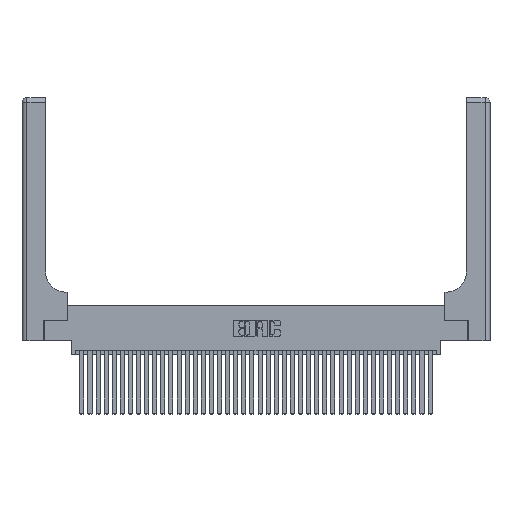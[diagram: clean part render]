
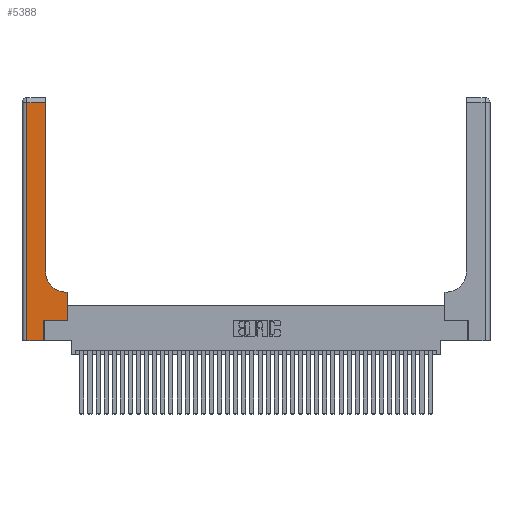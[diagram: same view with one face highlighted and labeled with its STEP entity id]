
A CAD part, top view. The second image highlights one B-rep face of the part: STEP entity #5388.
In plain terms, the highlighted planar face has unit normal (0, 0, 1).
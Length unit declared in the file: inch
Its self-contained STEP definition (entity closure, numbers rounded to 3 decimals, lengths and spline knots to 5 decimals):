
#55 = VERTEX_POINT ( 'NONE', #9593 ) ;
#679 = VERTEX_POINT ( 'NONE', #28018 ) ;
#1475 = VECTOR ( 'NONE', #24072, 39.37008 ) ;
#1845 = VERTEX_POINT ( 'NONE', #36134 ) ;
#2176 = VECTOR ( 'NONE', #4003, 39.37008 ) ;
#2212 = LINE ( 'NONE', #38274, #26557 ) ;
#4003 = DIRECTION ( 'NONE',  ( -1., 0., 0. ) ) ;
#5207 = ORIENTED_EDGE ( 'NONE', *, *, #17527, .T. ) ;
#5388 = ADVANCED_FACE ( 'NONE', ( #31855 ), #8118, .F. ) ;
#5506 = LINE ( 'NONE', #39268, #29762 ) ;
#7099 = VERTEX_POINT ( 'NONE', #28311 ) ;
#7922 = DIRECTION ( 'NONE',  ( 0., 1., 0. ) ) ;
#8118 = PLANE ( 'NONE',  #24441 ) ;
#8122 = ORIENTED_EDGE ( 'NONE', *, *, #33617, .T. ) ;
#8871 = CARTESIAN_POINT ( 'NONE',  ( 0.5415, 0.6, 0.37 ) ) ;
#9434 = DIRECTION ( 'NONE',  ( 0., -1., 0. ) ) ;
#9593 = CARTESIAN_POINT ( 'NONE',  ( 0.269, 0.25, 0.37 ) ) ;
#9673 = LINE ( 'NONE', #33059, #1475 ) ;
#10085 = DIRECTION ( 'NONE',  ( 0., 0., -1. ) ) ;
#10752 = DIRECTION ( 'NONE',  ( 0., 1., 0. ) ) ;
#11184 = DIRECTION ( 'NONE',  ( 0., 0., -1. ) ) ;
#11329 = LINE ( 'NONE', #19222, #2176 ) ;
#11651 = VERTEX_POINT ( 'NONE', #26555 ) ;
#12263 = CARTESIAN_POINT ( 'NONE',  ( 0.2915, 0.6, 0.37 ) ) ;
#12870 = CARTESIAN_POINT ( 'NONE',  ( 0.269, 0., 0.37 ) ) ;
#13168 = LINE ( 'NONE', #25882, #22160 ) ;
#13370 = ORIENTED_EDGE ( 'NONE', *, *, #27678, .T. ) ;
#14698 = VECTOR ( 'NONE', #33447, 39.37008 ) ;
#15318 = EDGE_CURVE ( 'NONE', #38560, #55, #30430, .T. ) ;
#15475 = CARTESIAN_POINT ( 'NONE',  ( 0.06, 3., 0.37 ) ) ;
#16254 = ORIENTED_EDGE ( 'NONE', *, *, #18850, .T. ) ;
#17061 = EDGE_CURVE ( 'NONE', #7099, #11651, #2212, .T. ) ;
#17527 = EDGE_CURVE ( 'NONE', #11651, #38305, #11329, .T. ) ;
#18408 = AXIS2_PLACEMENT_3D ( 'NONE', #28274, #10085, #31320 ) ;
#18850 = EDGE_CURVE ( 'NONE', #1845, #34125, #13168, .T. ) ;
#19222 = CARTESIAN_POINT ( 'NONE',  ( 0., 2.94, 0.37 ) ) ;
#19546 = ORIENTED_EDGE ( 'NONE', *, *, #15318, .T. ) ;
#20319 = EDGE_CURVE ( 'NONE', #32455, #7099, #24579, .T. ) ;
#21175 = DIRECTION ( 'NONE',  ( 1., 0., 0. ) ) ;
#22160 = VECTOR ( 'NONE', #10752, 39.37008 ) ;
#24072 = DIRECTION ( 'NONE',  ( 1., 0., 0. ) ) ;
#24441 = AXIS2_PLACEMENT_3D ( 'NONE', #29379, #11184, #32405 ) ;
#24579 = CIRCLE ( 'NONE', #18408, 0.25 ) ;
#25684 = VECTOR ( 'NONE', #9434, 39.37008 ) ;
#25751 = EDGE_CURVE ( 'NONE', #34125, #32455, #37878, .T. ) ;
#25882 = CARTESIAN_POINT ( 'NONE',  ( 0.5585, 0.25, 0.37 ) ) ;
#26324 = CARTESIAN_POINT ( 'NONE',  ( 0.5585, 0.6, 0.37 ) ) ;
#26555 = CARTESIAN_POINT ( 'NONE',  ( 0.2915, 2.94, 0.37 ) ) ;
#26557 = VECTOR ( 'NONE', #35392, 39.37008 ) ;
#26636 = LINE ( 'NONE', #15475, #25684 ) ;
#27144 = ORIENTED_EDGE ( 'NONE', *, *, #25751, .T. ) ;
#27678 = EDGE_CURVE ( 'NONE', #38305, #679, #26636, .T. ) ;
#28018 = CARTESIAN_POINT ( 'NONE',  ( 0.06, 0., 0.37 ) ) ;
#28274 = CARTESIAN_POINT ( 'NONE',  ( 0.5415, 0.85, 0.37 ) ) ;
#28311 = CARTESIAN_POINT ( 'NONE',  ( 0.2915, 0.85, 0.37 ) ) ;
#29175 = CARTESIAN_POINT ( 'NONE',  ( 0.269, 0., 0.37 ) ) ;
#29379 = CARTESIAN_POINT ( 'NONE',  ( 0., 3., 0.37 ) ) ;
#29499 = VECTOR ( 'NONE', #7922, 39.37008 ) ;
#29762 = VECTOR ( 'NONE', #21175, 39.37008 ) ;
#29996 = ORIENTED_EDGE ( 'NONE', *, *, #20319, .T. ) ;
#30430 = LINE ( 'NONE', #29175, #29499 ) ;
#31320 = DIRECTION ( 'NONE',  ( 1., 0., 0. ) ) ;
#31561 = EDGE_CURVE ( 'NONE', #679, #38560, #9673, .T. ) ;
#31855 = FACE_OUTER_BOUND ( 'NONE', #36016, .T. ) ;
#32405 = DIRECTION ( 'NONE',  ( -1., 0., 0. ) ) ;
#32455 = VERTEX_POINT ( 'NONE', #8871 ) ;
#33059 = CARTESIAN_POINT ( 'NONE',  ( 0., 0., 0.37 ) ) ;
#33447 = DIRECTION ( 'NONE',  ( -1., 0., 0. ) ) ;
#33617 = EDGE_CURVE ( 'NONE', #55, #1845, #5506, .T. ) ;
#34125 = VERTEX_POINT ( 'NONE', #26324 ) ;
#34646 = ORIENTED_EDGE ( 'NONE', *, *, #17061, .T. ) ;
#35392 = DIRECTION ( 'NONE',  ( 0., 1., 0. ) ) ;
#35761 = CARTESIAN_POINT ( 'NONE',  ( 0.06, 2.94, 0.37 ) ) ;
#36016 = EDGE_LOOP ( 'NONE', ( #34646, #5207, #13370, #36090, #19546, #8122, #16254, #27144, #29996 ) ) ;
#36090 = ORIENTED_EDGE ( 'NONE', *, *, #31561, .T. ) ;
#36134 = CARTESIAN_POINT ( 'NONE',  ( 0.5585, 0.25, 0.37 ) ) ;
#37878 = LINE ( 'NONE', #12263, #14698 ) ;
#38274 = CARTESIAN_POINT ( 'NONE',  ( 0.2915, 3., 0.37 ) ) ;
#38305 = VERTEX_POINT ( 'NONE', #35761 ) ;
#38560 = VERTEX_POINT ( 'NONE', #12870 ) ;
#39268 = CARTESIAN_POINT ( 'NONE',  ( 0.269, 0.25, 0.37 ) ) ;
